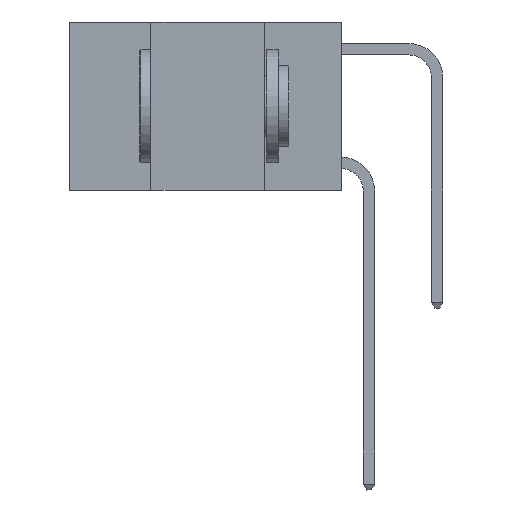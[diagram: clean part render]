
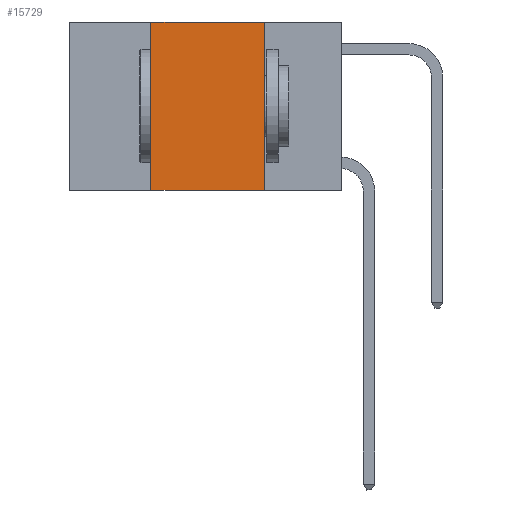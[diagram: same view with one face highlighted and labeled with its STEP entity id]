
A CAD part, left-side view. The second image highlights one B-rep face of the part: STEP entity #15729.
In plain terms, the highlighted planar face has unit normal (-1, 0, 0).
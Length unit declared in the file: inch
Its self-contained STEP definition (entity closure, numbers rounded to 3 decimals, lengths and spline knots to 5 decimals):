
#797 = VERTEX_POINT ( 'NONE', #2262 ) ;
#992 = AXIS2_PLACEMENT_3D ( 'NONE', #14582, #5393, #14680 ) ;
#1984 = EDGE_CURVE ( 'NONE', #8811, #2452, #18054, .T. ) ;
#2093 = EDGE_LOOP ( 'NONE', ( #8327, #19401, #17978, #2524 ) ) ;
#2262 = CARTESIAN_POINT ( 'NONE',  ( 0., 0.17, -0.37 ) ) ;
#2452 = VERTEX_POINT ( 'NONE', #13434 ) ;
#2502 = LINE ( 'NONE', #8179, #11775 ) ;
#2524 = ORIENTED_EDGE ( 'NONE', *, *, #15369, .T. ) ;
#2764 = CARTESIAN_POINT ( 'NONE',  ( 0., 0.42, -0.37 ) ) ;
#2829 = DIRECTION ( 'NONE',  ( 0., -1., 0. ) ) ;
#5383 = LINE ( 'NONE', #11031, #13538 ) ;
#5393 = DIRECTION ( 'NONE',  ( 1., 0., 0. ) ) ;
#7173 = DIRECTION ( 'NONE',  ( 0., 0., 1. ) ) ;
#7652 = VERTEX_POINT ( 'NONE', #9560 ) ;
#8179 = CARTESIAN_POINT ( 'NONE',  ( 0., 0.17, 0. ) ) ;
#8327 = ORIENTED_EDGE ( 'NONE', *, *, #17522, .F. ) ;
#8811 = VERTEX_POINT ( 'NONE', #2764 ) ;
#9560 = CARTESIAN_POINT ( 'NONE',  ( 0., 0.17, 0. ) ) ;
#9766 = DIRECTION ( 'NONE',  ( 0., 0., -1. ) ) ;
#10743 = LINE ( 'NONE', #13701, #11101 ) ;
#11031 = CARTESIAN_POINT ( 'NONE',  ( 0., 0.6, 0. ) ) ;
#11101 = VECTOR ( 'NONE', #2829, 39.37008 ) ;
#11226 = DIRECTION ( 'NONE',  ( 0., -1., 0. ) ) ;
#11415 = EDGE_CURVE ( 'NONE', #2452, #7652, #5383, .T. ) ;
#11775 = VECTOR ( 'NONE', #9766, 39.37008 ) ;
#13434 = CARTESIAN_POINT ( 'NONE',  ( 0., 0.42, 0. ) ) ;
#13538 = VECTOR ( 'NONE', #11226, 39.37008 ) ;
#13701 = CARTESIAN_POINT ( 'NONE',  ( 0., 0.6, -0.37 ) ) ;
#14392 = FACE_OUTER_BOUND ( 'NONE', #2093, .T. ) ;
#14582 = CARTESIAN_POINT ( 'NONE',  ( 0., 0.6, 0. ) ) ;
#14680 = DIRECTION ( 'NONE',  ( 0., 0., -1. ) ) ;
#14882 = CARTESIAN_POINT ( 'NONE',  ( 0., 0.42, 0. ) ) ;
#15369 = EDGE_CURVE ( 'NONE', #8811, #797, #10743, .T. ) ;
#15729 = ADVANCED_FACE ( 'NONE', ( #14392 ), #19237, .F. ) ;
#17522 = EDGE_CURVE ( 'NONE', #7652, #797, #2502, .T. ) ;
#17978 = ORIENTED_EDGE ( 'NONE', *, *, #1984, .F. ) ;
#18054 = LINE ( 'NONE', #14882, #18916 ) ;
#18916 = VECTOR ( 'NONE', #7173, 39.37008 ) ;
#19237 = PLANE ( 'NONE',  #992 ) ;
#19401 = ORIENTED_EDGE ( 'NONE', *, *, #11415, .F. ) ;
